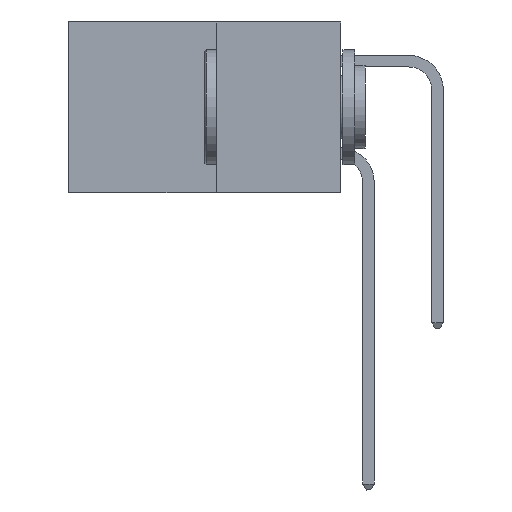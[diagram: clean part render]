
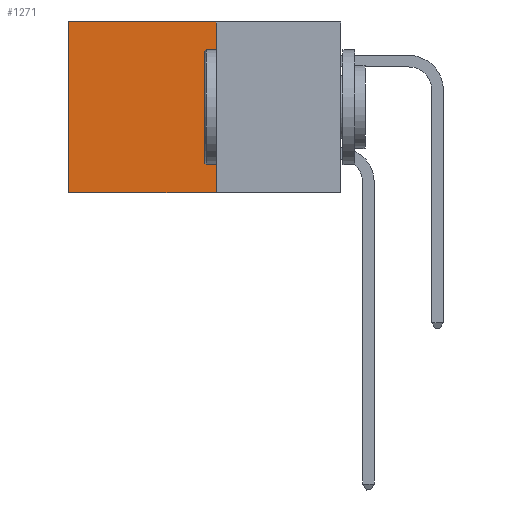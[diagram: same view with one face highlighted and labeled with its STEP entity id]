
A CAD part, left-side view. The second image highlights one B-rep face of the part: STEP entity #1271.
In plain terms, the highlighted planar face has unit normal (-1, 0, 0).
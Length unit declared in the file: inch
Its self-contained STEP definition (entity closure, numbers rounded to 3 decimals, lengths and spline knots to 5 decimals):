
#105 = DIRECTION ( 'NONE',  ( 0., 0., -1. ) ) ;
#874 = AXIS2_PLACEMENT_3D ( 'NONE', #11864, #18935, #15795 ) ;
#1269 = CARTESIAN_POINT ( 'NONE',  ( 0.277, 0.27, -0.37 ) ) ;
#1271 = ADVANCED_FACE ( 'NONE', ( #15211 ), #9401, .F. ) ;
#1638 = LINE ( 'NONE', #5717, #16843 ) ;
#3347 = ORIENTED_EDGE ( 'NONE', *, *, #9002, .T. ) ;
#5196 = ORIENTED_EDGE ( 'NONE', *, *, #17839, .T. ) ;
#5507 = DIRECTION ( 'NONE',  ( 0., 0., -1. ) ) ;
#5607 = DIRECTION ( 'NONE',  ( 0., 1., 0. ) ) ;
#5717 = CARTESIAN_POINT ( 'NONE',  ( 0.277, 0.27, -0.37 ) ) ;
#5902 = LINE ( 'NONE', #15136, #17238 ) ;
#6042 = VERTEX_POINT ( 'NONE', #16537 ) ;
#6854 = VECTOR ( 'NONE', #105, 39.37008 ) ;
#7302 = EDGE_CURVE ( 'NONE', #6042, #16441, #1638, .T. ) ;
#7423 = CARTESIAN_POINT ( 'NONE',  ( 0.277, 0.59, -0.37 ) ) ;
#7706 = DIRECTION ( 'NONE',  ( 0., 1., 0. ) ) ;
#8823 = CARTESIAN_POINT ( 'NONE',  ( 0.277, 0.27, 0. ) ) ;
#9002 = EDGE_CURVE ( 'NONE', #6042, #13821, #11232, .T. ) ;
#9401 = PLANE ( 'NONE',  #874 ) ;
#9878 = LINE ( 'NONE', #7423, #6854 ) ;
#10243 = CARTESIAN_POINT ( 'NONE',  ( 0.277, 0.59, -0.37 ) ) ;
#10786 = VECTOR ( 'NONE', #5607, 39.37008 ) ;
#10896 = ORIENTED_EDGE ( 'NONE', *, *, #7302, .F. ) ;
#11232 = LINE ( 'NONE', #8823, #10786 ) ;
#11860 = EDGE_CURVE ( 'NONE', #16441, #17090, #5902, .T. ) ;
#11864 = CARTESIAN_POINT ( 'NONE',  ( 0.277, 0.27, -0.37 ) ) ;
#12550 = EDGE_LOOP ( 'NONE', ( #5196, #13956, #10896, #3347 ) ) ;
#13821 = VERTEX_POINT ( 'NONE', #15146 ) ;
#13956 = ORIENTED_EDGE ( 'NONE', *, *, #11860, .F. ) ;
#15136 = CARTESIAN_POINT ( 'NONE',  ( 0.277, 0.27, -0.37 ) ) ;
#15146 = CARTESIAN_POINT ( 'NONE',  ( 0.277, 0.59, 0. ) ) ;
#15211 = FACE_OUTER_BOUND ( 'NONE', #12550, .T. ) ;
#15795 = DIRECTION ( 'NONE',  ( 0., 0., -1. ) ) ;
#16441 = VERTEX_POINT ( 'NONE', #1269 ) ;
#16537 = CARTESIAN_POINT ( 'NONE',  ( 0.277, 0.27, 0. ) ) ;
#16843 = VECTOR ( 'NONE', #5507, 39.37008 ) ;
#17090 = VERTEX_POINT ( 'NONE', #10243 ) ;
#17238 = VECTOR ( 'NONE', #7706, 39.37008 ) ;
#17839 = EDGE_CURVE ( 'NONE', #13821, #17090, #9878, .T. ) ;
#18935 = DIRECTION ( 'NONE',  ( 1., 0., 0. ) ) ;
